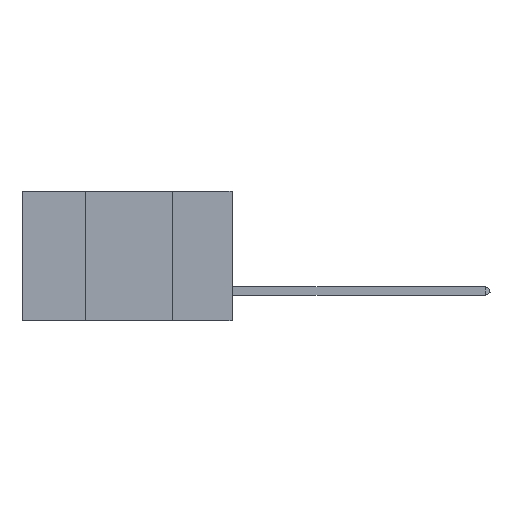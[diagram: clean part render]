
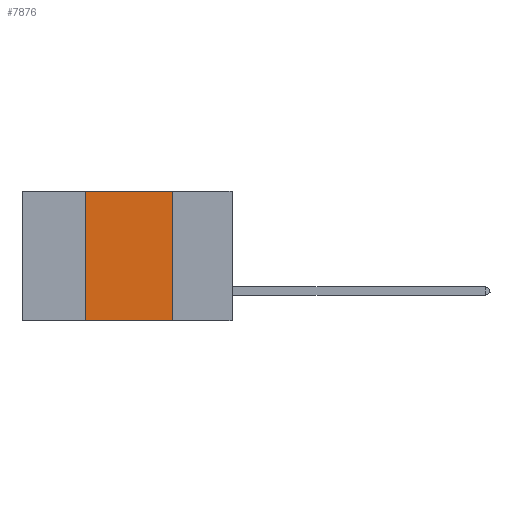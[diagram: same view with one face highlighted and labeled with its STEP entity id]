
A CAD part, left-side view. The second image highlights one B-rep face of the part: STEP entity #7876.
In plain terms, the highlighted planar face has unit normal (-1, 0, 0).
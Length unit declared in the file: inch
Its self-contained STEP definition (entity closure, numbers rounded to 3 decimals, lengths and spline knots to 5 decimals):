
#1271 = CARTESIAN_POINT ( 'NONE',  ( 0., 0.17, 0. ) ) ;
#1621 = CARTESIAN_POINT ( 'NONE',  ( 0., 0.42, -0.37 ) ) ;
#2299 = EDGE_CURVE ( 'NONE', #2589, #12230, #18258, .T. ) ;
#2589 = VERTEX_POINT ( 'NONE', #1621 ) ;
#3046 = PLANE ( 'NONE',  #19346 ) ;
#3400 = FACE_OUTER_BOUND ( 'NONE', #14483, .T. ) ;
#3560 = VECTOR ( 'NONE', #16472, 39.37008 ) ;
#3611 = DIRECTION ( 'NONE',  ( 0., -1., 0. ) ) ;
#4437 = LINE ( 'NONE', #19584, #12123 ) ;
#4553 = CARTESIAN_POINT ( 'NONE',  ( 0., 0.6, 0. ) ) ;
#5107 = LINE ( 'NONE', #19725, #3560 ) ;
#5287 = VERTEX_POINT ( 'NONE', #1271 ) ;
#6388 = DIRECTION ( 'NONE',  ( 0., 0., -1. ) ) ;
#6793 = CARTESIAN_POINT ( 'NONE',  ( 0., 0.6, -0.37 ) ) ;
#7022 = LINE ( 'NONE', #7974, #12162 ) ;
#7876 = ADVANCED_FACE ( 'NONE', ( #3400 ), #3046, .F. ) ;
#7974 = CARTESIAN_POINT ( 'NONE',  ( 0., 0.42, 0. ) ) ;
#8520 = ORIENTED_EDGE ( 'NONE', *, *, #19776, .F. ) ;
#10125 = CARTESIAN_POINT ( 'NONE',  ( 0., 0.42, 0. ) ) ;
#10138 = VERTEX_POINT ( 'NONE', #10125 ) ;
#10402 = ORIENTED_EDGE ( 'NONE', *, *, #18810, .F. ) ;
#12123 = VECTOR ( 'NONE', #13176, 39.37008 ) ;
#12162 = VECTOR ( 'NONE', #19411, 39.37008 ) ;
#12230 = VERTEX_POINT ( 'NONE', #15199 ) ;
#13176 = DIRECTION ( 'NONE',  ( 0., 0., -1. ) ) ;
#13936 = VECTOR ( 'NONE', #3611, 39.37008 ) ;
#14231 = ORIENTED_EDGE ( 'NONE', *, *, #16647, .F. ) ;
#14327 = DIRECTION ( 'NONE',  ( 1., 0., 0. ) ) ;
#14483 = EDGE_LOOP ( 'NONE', ( #14231, #10402, #8520, #19197 ) ) ;
#15199 = CARTESIAN_POINT ( 'NONE',  ( 0., 0.17, -0.37 ) ) ;
#16472 = DIRECTION ( 'NONE',  ( 0., -1., 0. ) ) ;
#16647 = EDGE_CURVE ( 'NONE', #5287, #12230, #4437, .T. ) ;
#18258 = LINE ( 'NONE', #6793, #13936 ) ;
#18810 = EDGE_CURVE ( 'NONE', #10138, #5287, #5107, .T. ) ;
#19197 = ORIENTED_EDGE ( 'NONE', *, *, #2299, .T. ) ;
#19346 = AXIS2_PLACEMENT_3D ( 'NONE', #4553, #14327, #6388 ) ;
#19411 = DIRECTION ( 'NONE',  ( 0., 0., 1. ) ) ;
#19584 = CARTESIAN_POINT ( 'NONE',  ( 0., 0.17, 0. ) ) ;
#19725 = CARTESIAN_POINT ( 'NONE',  ( 0., 0.6, 0. ) ) ;
#19776 = EDGE_CURVE ( 'NONE', #2589, #10138, #7022, .T. ) ;
